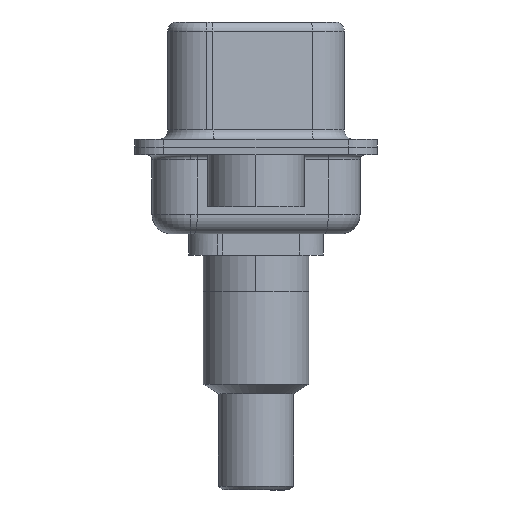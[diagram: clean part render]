
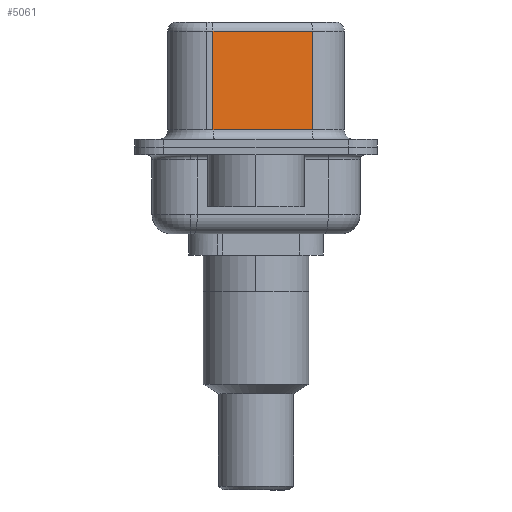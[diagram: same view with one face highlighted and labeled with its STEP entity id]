
A CAD part, left-side view. The second image highlights one B-rep face of the part: STEP entity #5061.
In plain terms, the highlighted planar face has unit normal (-0.985, -0.174, 0).
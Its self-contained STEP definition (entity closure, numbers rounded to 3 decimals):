
#324 = AXIS2_PLACEMENT_3D ( 'NONE', #19010, #2612, #13071 ) ;
#468 = VECTOR ( 'NONE', #18206, 1000. ) ;
#901 = CARTESIAN_POINT ( 'NONE',  ( 3.655, 2.233, 6.52 ) ) ;
#1059 = CARTESIAN_POINT ( 'NONE',  ( 3.655, 2.233, 6.02 ) ) ;
#1103 = ORIENTED_EDGE ( 'NONE', *, *, #5476, .T. ) ;
#1464 = LINE ( 'NONE', #2731, #9394 ) ;
#1807 = CARTESIAN_POINT ( 'NONE',  ( 3.655, 2.233, 0.9 ) ) ;
#2400 = DIRECTION ( 'NONE',  ( 0., 0., -1. ) ) ;
#2612 = DIRECTION ( 'NONE',  ( 0.985, 0.174, 0. ) ) ;
#2626 = ORIENTED_EDGE ( 'NONE', *, *, #9307, .T. ) ;
#2731 = CARTESIAN_POINT ( 'NONE',  ( 4.565, -2.927, 0.9 ) ) ;
#3241 = CARTESIAN_POINT ( 'NONE',  ( 4.565, -2.927, 6.02 ) ) ;
#4069 = EDGE_CURVE ( 'NONE', #17928, #4935, #13141, .T. ) ;
#4423 = LINE ( 'NONE', #3241, #468 ) ;
#4702 = ORIENTED_EDGE ( 'NONE', *, *, #4069, .F. ) ;
#4935 = VERTEX_POINT ( 'NONE', #12757 ) ;
#5061 = ADVANCED_FACE ( 'NONE', ( #9107 ), #14494, .F. ) ;
#5476 = EDGE_CURVE ( 'NONE', #10903, #8688, #18012, .T. ) ;
#6086 = VECTOR ( 'NONE', #2400, 1000. ) ;
#6595 = CARTESIAN_POINT ( 'NONE',  ( 4.565, -2.927, 6.52 ) ) ;
#8688 = VERTEX_POINT ( 'NONE', #1807 ) ;
#9107 = FACE_OUTER_BOUND ( 'NONE', #13566, .T. ) ;
#9307 = EDGE_CURVE ( 'NONE', #8688, #4935, #1464, .T. ) ;
#9394 = VECTOR ( 'NONE', #13216, 1000. ) ;
#10751 = ORIENTED_EDGE ( 'NONE', *, *, #12527, .T. ) ;
#10903 = VERTEX_POINT ( 'NONE', #1059 ) ;
#12206 = VECTOR ( 'NONE', #16532, 1000. ) ;
#12527 = EDGE_CURVE ( 'NONE', #17928, #10903, #4423, .T. ) ;
#12757 = CARTESIAN_POINT ( 'NONE',  ( 4.565, -2.927, 0.9 ) ) ;
#13071 = DIRECTION ( 'NONE',  ( -0.174, 0.985, 0. ) ) ;
#13141 = LINE ( 'NONE', #6595, #12206 ) ;
#13216 = DIRECTION ( 'NONE',  ( 0.174, -0.985, 0. ) ) ;
#13566 = EDGE_LOOP ( 'NONE', ( #4702, #10751, #1103, #2626 ) ) ;
#14494 = PLANE ( 'NONE',  #324 ) ;
#14869 = CARTESIAN_POINT ( 'NONE',  ( 4.565, -2.927, 6.02 ) ) ;
#16532 = DIRECTION ( 'NONE',  ( 0., 0., -1. ) ) ;
#17928 = VERTEX_POINT ( 'NONE', #14869 ) ;
#18012 = LINE ( 'NONE', #901, #6086 ) ;
#18206 = DIRECTION ( 'NONE',  ( -0.174, 0.985, 0. ) ) ;
#19010 = CARTESIAN_POINT ( 'NONE',  ( 4.565, -2.927, 6.52 ) ) ;
